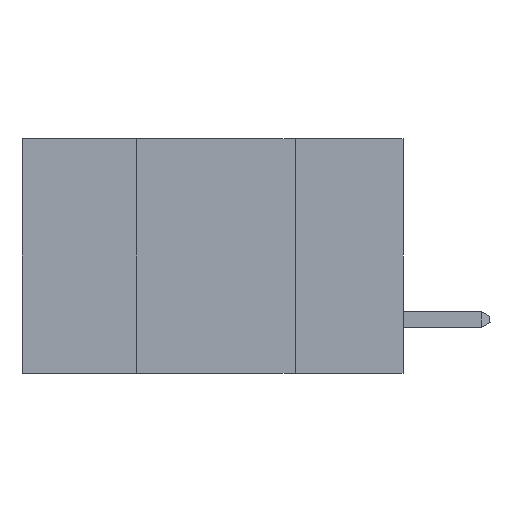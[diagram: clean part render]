
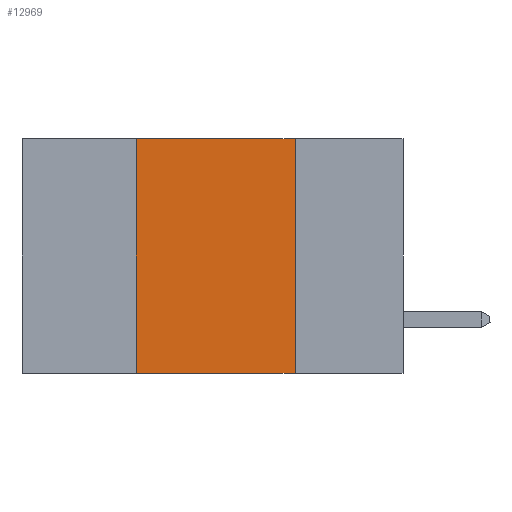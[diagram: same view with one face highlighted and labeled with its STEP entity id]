
A CAD part, left-side view. The second image highlights one B-rep face of the part: STEP entity #12969.
In plain terms, the highlighted planar face has unit normal (-1, 0, 0).
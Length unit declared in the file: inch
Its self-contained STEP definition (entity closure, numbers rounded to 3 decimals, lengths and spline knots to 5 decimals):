
#519 = DIRECTION ( 'NONE',  ( 0., -1., 0. ) ) ;
#545 = DIRECTION ( 'NONE',  ( 0., 0., 1. ) ) ;
#978 = EDGE_CURVE ( 'NONE', #12603, #8641, #12351, .T. ) ;
#1011 = CARTESIAN_POINT ( 'NONE',  ( 0., 0.42, 0. ) ) ;
#1051 = VECTOR ( 'NONE', #519, 39.37008 ) ;
#1278 = EDGE_LOOP ( 'NONE', ( #13067, #1638, #6960, #8234 ) ) ;
#1638 = ORIENTED_EDGE ( 'NONE', *, *, #978, .F. ) ;
#1783 = CARTESIAN_POINT ( 'NONE',  ( 0., 0.17, 0. ) ) ;
#1877 = VECTOR ( 'NONE', #3778, 39.37008 ) ;
#2112 = LINE ( 'NONE', #7580, #11505 ) ;
#2856 = CARTESIAN_POINT ( 'NONE',  ( 0., 0.6, -0.37 ) ) ;
#3031 = VECTOR ( 'NONE', #9020, 39.37008 ) ;
#3629 = PLANE ( 'NONE',  #12053 ) ;
#3778 = DIRECTION ( 'NONE',  ( 0., 0., -1. ) ) ;
#4081 = CARTESIAN_POINT ( 'NONE',  ( 0., 0.17, -0.37 ) ) ;
#4306 = EDGE_CURVE ( 'NONE', #8508, #12603, #2112, .T. ) ;
#4526 = CARTESIAN_POINT ( 'NONE',  ( 0., 0.42, -0.37 ) ) ;
#4648 = DIRECTION ( 'NONE',  ( 0., 0., -1. ) ) ;
#4687 = CARTESIAN_POINT ( 'NONE',  ( 0., 0.6, 0. ) ) ;
#5334 = LINE ( 'NONE', #1783, #1877 ) ;
#6284 = EDGE_CURVE ( 'NONE', #8641, #11221, #5334, .T. ) ;
#6960 = ORIENTED_EDGE ( 'NONE', *, *, #4306, .F. ) ;
#7357 = FACE_OUTER_BOUND ( 'NONE', #1278, .T. ) ;
#7580 = CARTESIAN_POINT ( 'NONE',  ( 0., 0.42, 0. ) ) ;
#8234 = ORIENTED_EDGE ( 'NONE', *, *, #9339, .T. ) ;
#8508 = VERTEX_POINT ( 'NONE', #4526 ) ;
#8641 = VERTEX_POINT ( 'NONE', #8892 ) ;
#8892 = CARTESIAN_POINT ( 'NONE',  ( 0., 0.17, 0. ) ) ;
#9020 = DIRECTION ( 'NONE',  ( 0., -1., 0. ) ) ;
#9339 = EDGE_CURVE ( 'NONE', #8508, #11221, #12456, .T. ) ;
#10830 = DIRECTION ( 'NONE',  ( 1., 0., 0. ) ) ;
#11221 = VERTEX_POINT ( 'NONE', #4081 ) ;
#11505 = VECTOR ( 'NONE', #545, 39.37008 ) ;
#11853 = CARTESIAN_POINT ( 'NONE',  ( 0., 0.6, 0. ) ) ;
#12053 = AXIS2_PLACEMENT_3D ( 'NONE', #4687, #10830, #4648 ) ;
#12351 = LINE ( 'NONE', #11853, #1051 ) ;
#12456 = LINE ( 'NONE', #2856, #3031 ) ;
#12603 = VERTEX_POINT ( 'NONE', #1011 ) ;
#12969 = ADVANCED_FACE ( 'NONE', ( #7357 ), #3629, .F. ) ;
#13067 = ORIENTED_EDGE ( 'NONE', *, *, #6284, .F. ) ;
